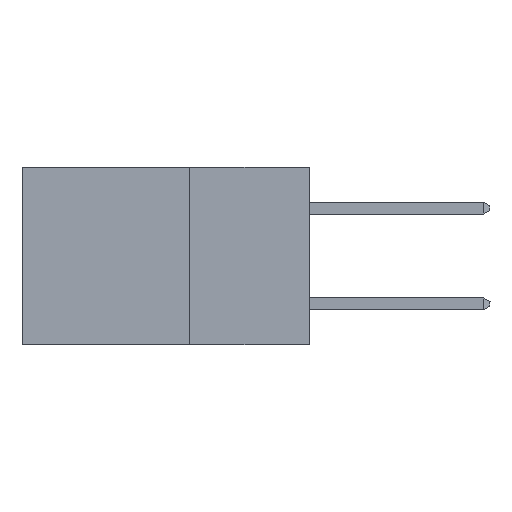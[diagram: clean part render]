
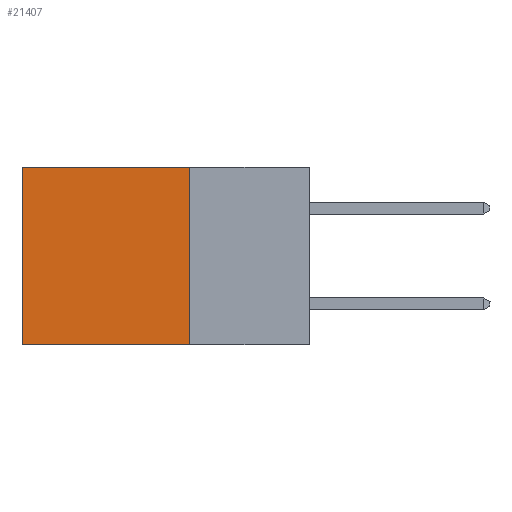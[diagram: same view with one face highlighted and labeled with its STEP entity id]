
A CAD part, left-side view. The second image highlights one B-rep face of the part: STEP entity #21407.
In plain terms, the highlighted planar face has unit normal (-1, 0, 0).
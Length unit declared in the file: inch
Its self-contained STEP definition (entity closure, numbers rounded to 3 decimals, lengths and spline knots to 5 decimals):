
#829 = EDGE_CURVE ( 'NONE', #2998, #10618, #11606, .T. ) ;
#2444 = PLANE ( 'NONE',  #12415 ) ;
#2884 = CARTESIAN_POINT ( 'NONE',  ( 0.2875, 0.25, -0.37 ) ) ;
#2998 = VERTEX_POINT ( 'NONE', #12968 ) ;
#3477 = VECTOR ( 'NONE', #30899, 39.37008 ) ;
#3861 = ORIENTED_EDGE ( 'NONE', *, *, #829, .F. ) ;
#4679 = ORIENTED_EDGE ( 'NONE', *, *, #18407, .F. ) ;
#5140 = DIRECTION ( 'NONE',  ( 0., 0., -1. ) ) ;
#5503 = LINE ( 'NONE', #20250, #29196 ) ;
#7180 = EDGE_LOOP ( 'NONE', ( #15162, #4679, #3861, #35168 ) ) ;
#7925 = CARTESIAN_POINT ( 'NONE',  ( 0.2875, 0.25, 0. ) ) ;
#9178 = LINE ( 'NONE', #2884, #3477 ) ;
#10618 = VERTEX_POINT ( 'NONE', #35248 ) ;
#10934 = CARTESIAN_POINT ( 'NONE',  ( 0.2875, 0.25, 0. ) ) ;
#10973 = DIRECTION ( 'NONE',  ( 1., 0., 0. ) ) ;
#11606 = LINE ( 'NONE', #10934, #19571 ) ;
#12415 = AXIS2_PLACEMENT_3D ( 'NONE', #7925, #10973, #5140 ) ;
#12942 = LINE ( 'NONE', #29493, #13819 ) ;
#12968 = CARTESIAN_POINT ( 'NONE',  ( 0.2875, 0.25, 0. ) ) ;
#13819 = VECTOR ( 'NONE', #15522, 39.37008 ) ;
#14720 = DIRECTION ( 'NONE',  ( 0., 1., 0. ) ) ;
#15162 = ORIENTED_EDGE ( 'NONE', *, *, #29877, .T. ) ;
#15522 = DIRECTION ( 'NONE',  ( 0., 0., -1. ) ) ;
#16015 = FACE_OUTER_BOUND ( 'NONE', #7180, .T. ) ;
#16329 = VERTEX_POINT ( 'NONE', #32541 ) ;
#18407 = EDGE_CURVE ( 'NONE', #10618, #33156, #9178, .T. ) ;
#19571 = VECTOR ( 'NONE', #19587, 39.37008 ) ;
#19587 = DIRECTION ( 'NONE',  ( 0., 0., -1. ) ) ;
#20250 = CARTESIAN_POINT ( 'NONE',  ( 0.2875, 0.25, 0. ) ) ;
#20975 = EDGE_CURVE ( 'NONE', #2998, #16329, #5503, .T. ) ;
#21407 = ADVANCED_FACE ( 'NONE', ( #16015 ), #2444, .F. ) ;
#29196 = VECTOR ( 'NONE', #14720, 39.37008 ) ;
#29493 = CARTESIAN_POINT ( 'NONE',  ( 0.2875, 0.6, 0. ) ) ;
#29877 = EDGE_CURVE ( 'NONE', #16329, #33156, #12942, .T. ) ;
#30899 = DIRECTION ( 'NONE',  ( 0., 1., 0. ) ) ;
#32541 = CARTESIAN_POINT ( 'NONE',  ( 0.2875, 0.6, 0. ) ) ;
#33156 = VERTEX_POINT ( 'NONE', #34845 ) ;
#34845 = CARTESIAN_POINT ( 'NONE',  ( 0.2875, 0.6, -0.37 ) ) ;
#35168 = ORIENTED_EDGE ( 'NONE', *, *, #20975, .T. ) ;
#35248 = CARTESIAN_POINT ( 'NONE',  ( 0.2875, 0.25, -0.37 ) ) ;
